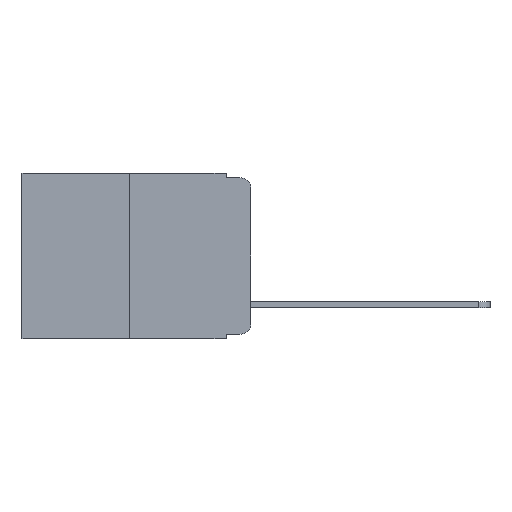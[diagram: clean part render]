
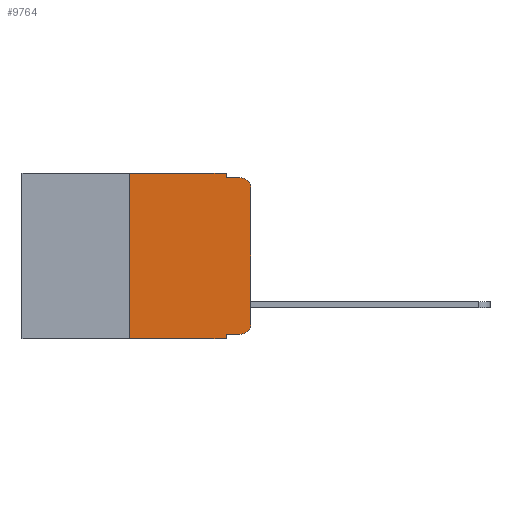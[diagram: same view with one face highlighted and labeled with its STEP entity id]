
A CAD part, left-side view. The second image highlights one B-rep face of the part: STEP entity #9764.
In plain terms, the highlighted planar face has unit normal (-1, 0, 0).
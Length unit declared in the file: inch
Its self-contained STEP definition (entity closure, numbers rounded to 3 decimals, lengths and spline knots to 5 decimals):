
#75 = VECTOR ( 'NONE', #4542, 39.37008 ) ;
#88 = CARTESIAN_POINT ( 'NONE',  ( 0., 0.473, -0.343 ) ) ;
#318 = CARTESIAN_POINT ( 'NONE',  ( 0., 0.02, -0.313 ) ) ;
#416 = ORIENTED_EDGE ( 'NONE', *, *, #10914, .T. ) ;
#684 = CARTESIAN_POINT ( 'NONE',  ( 0., 0.051, -0.333 ) ) ;
#834 = ORIENTED_EDGE ( 'NONE', *, *, #6526, .F. ) ;
#905 = VERTEX_POINT ( 'NONE', #13053 ) ;
#1074 = CIRCLE ( 'NONE', #1084, 0.02 ) ;
#1084 = AXIS2_PLACEMENT_3D ( 'NONE', #12921, #11837, #14115 ) ;
#1215 = LINE ( 'NONE', #8678, #2797 ) ;
#1223 = EDGE_CURVE ( 'NONE', #905, #7131, #1074, .T. ) ;
#1381 = ORIENTED_EDGE ( 'NONE', *, *, #7744, .T. ) ;
#1488 = CARTESIAN_POINT ( 'NONE',  ( 0., 0.473, 0. ) ) ;
#1645 = ORIENTED_EDGE ( 'NONE', *, *, #5811, .T. ) ;
#1753 = ORIENTED_EDGE ( 'NONE', *, *, #9422, .F. ) ;
#1997 = ORIENTED_EDGE ( 'NONE', *, *, #14435, .T. ) ;
#2050 = VECTOR ( 'NONE', #10989, 39.37008 ) ;
#2220 = VERTEX_POINT ( 'NONE', #3481 ) ;
#2292 = DIRECTION ( 'NONE',  ( 0., -1., 0. ) ) ;
#2363 = VECTOR ( 'NONE', #7740, 39.37008 ) ;
#2479 = VECTOR ( 'NONE', #11544, 39.37008 ) ;
#2704 = CARTESIAN_POINT ( 'NONE',  ( 0., 0.25, -0.343 ) ) ;
#2797 = VECTOR ( 'NONE', #2292, 39.37008 ) ;
#3016 = LINE ( 'NONE', #5893, #9059 ) ;
#3084 = LINE ( 'NONE', #88, #75 ) ;
#3362 = ORIENTED_EDGE ( 'NONE', *, *, #3996, .F. ) ;
#3481 = CARTESIAN_POINT ( 'NONE',  ( 0., 0., -0.313 ) ) ;
#3996 = EDGE_CURVE ( 'NONE', #14261, #7131, #1215, .T. ) ;
#4349 = CARTESIAN_POINT ( 'NONE',  ( 0., 0.051, 0. ) ) ;
#4473 = ORIENTED_EDGE ( 'NONE', *, *, #9541, .F. ) ;
#4505 = LINE ( 'NONE', #684, #2050 ) ;
#4542 = DIRECTION ( 'NONE',  ( 0., -1., 0. ) ) ;
#4592 = CARTESIAN_POINT ( 'NONE',  ( 0., 0., 0. ) ) ;
#4888 = CARTESIAN_POINT ( 'NONE',  ( 0., 0.02, -0.01 ) ) ;
#4974 = CIRCLE ( 'NONE', #5290, 0.02 ) ;
#5266 = CARTESIAN_POINT ( 'NONE',  ( 0., 0.25, 0. ) ) ;
#5290 = AXIS2_PLACEMENT_3D ( 'NONE', #318, #8265, #10581 ) ;
#5325 = LINE ( 'NONE', #5266, #12608 ) ;
#5431 = DIRECTION ( 'NONE',  ( 0., 0., -1. ) ) ;
#5488 = LINE ( 'NONE', #4592, #2479 ) ;
#5530 = CARTESIAN_POINT ( 'NONE',  ( 0., 0.051, 0. ) ) ;
#5811 = EDGE_CURVE ( 'NONE', #13908, #14369, #3084, .T. ) ;
#5893 = CARTESIAN_POINT ( 'NONE',  ( 0., 0.473, 0. ) ) ;
#5926 = DIRECTION ( 'NONE',  ( 0., 0., -1. ) ) ;
#6000 = ORIENTED_EDGE ( 'NONE', *, *, #1223, .T. ) ;
#6168 = CARTESIAN_POINT ( 'NONE',  ( 0., 0.051, -0.01 ) ) ;
#6480 = CARTESIAN_POINT ( 'NONE',  ( 0., 0.051, -0.343 ) ) ;
#6526 = EDGE_CURVE ( 'NONE', #8021, #14369, #8567, .T. ) ;
#6601 = VECTOR ( 'NONE', #5431, 39.37008 ) ;
#7131 = VERTEX_POINT ( 'NONE', #4888 ) ;
#7414 = VERTEX_POINT ( 'NONE', #5530 ) ;
#7740 = DIRECTION ( 'NONE',  ( 0., 0., -1. ) ) ;
#7744 = EDGE_CURVE ( 'NONE', #12663, #2220, #4974, .T. ) ;
#7776 = ORIENTED_EDGE ( 'NONE', *, *, #12307, .F. ) ;
#7909 = AXIS2_PLACEMENT_3D ( 'NONE', #1488, #13920, #5926 ) ;
#8021 = VERTEX_POINT ( 'NONE', #9987 ) ;
#8265 = DIRECTION ( 'NONE',  ( -1., 0., 0. ) ) ;
#8567 = LINE ( 'NONE', #10091, #6601 ) ;
#8678 = CARTESIAN_POINT ( 'NONE',  ( 0., 0.051, -0.01 ) ) ;
#9059 = VECTOR ( 'NONE', #13938, 39.37008 ) ;
#9078 = VERTEX_POINT ( 'NONE', #14689 ) ;
#9282 = LINE ( 'NONE', #4349, #2363 ) ;
#9390 = PLANE ( 'NONE',  #7909 ) ;
#9422 = EDGE_CURVE ( 'NONE', #13908, #9078, #5325, .T. ) ;
#9541 = EDGE_CURVE ( 'NONE', #9078, #7414, #3016, .T. ) ;
#9764 = ADVANCED_FACE ( 'NONE', ( #10996 ), #9390, .F. ) ;
#9987 = CARTESIAN_POINT ( 'NONE',  ( 0., 0.051, -0.333 ) ) ;
#10091 = CARTESIAN_POINT ( 'NONE',  ( 0., 0.051, 0. ) ) ;
#10581 = DIRECTION ( 'NONE',  ( 0., 0., -1. ) ) ;
#10783 = DIRECTION ( 'NONE',  ( 0., 0., 1. ) ) ;
#10914 = EDGE_CURVE ( 'NONE', #2220, #905, #5488, .T. ) ;
#10989 = DIRECTION ( 'NONE',  ( 0., -1., 0. ) ) ;
#10996 = FACE_OUTER_BOUND ( 'NONE', #13509, .T. ) ;
#11544 = DIRECTION ( 'NONE',  ( 0., 0., 1. ) ) ;
#11837 = DIRECTION ( 'NONE',  ( -1., 0., 0. ) ) ;
#12307 = EDGE_CURVE ( 'NONE', #7414, #14261, #9282, .T. ) ;
#12608 = VECTOR ( 'NONE', #10783, 39.37008 ) ;
#12663 = VERTEX_POINT ( 'NONE', #12802 ) ;
#12802 = CARTESIAN_POINT ( 'NONE',  ( 0., 0.02, -0.333 ) ) ;
#12921 = CARTESIAN_POINT ( 'NONE',  ( 0., 0.02, -0.03 ) ) ;
#13053 = CARTESIAN_POINT ( 'NONE',  ( 0., 0., -0.03 ) ) ;
#13509 = EDGE_LOOP ( 'NONE', ( #416, #6000, #3362, #7776, #4473, #1753, #1645, #834, #1997, #1381 ) ) ;
#13908 = VERTEX_POINT ( 'NONE', #2704 ) ;
#13920 = DIRECTION ( 'NONE',  ( 1., 0., 0. ) ) ;
#13938 = DIRECTION ( 'NONE',  ( 0., -1., 0. ) ) ;
#14115 = DIRECTION ( 'NONE',  ( 0., 0., -1. ) ) ;
#14261 = VERTEX_POINT ( 'NONE', #6168 ) ;
#14369 = VERTEX_POINT ( 'NONE', #6480 ) ;
#14435 = EDGE_CURVE ( 'NONE', #8021, #12663, #4505, .T. ) ;
#14689 = CARTESIAN_POINT ( 'NONE',  ( 0., 0.25, 0. ) ) ;
